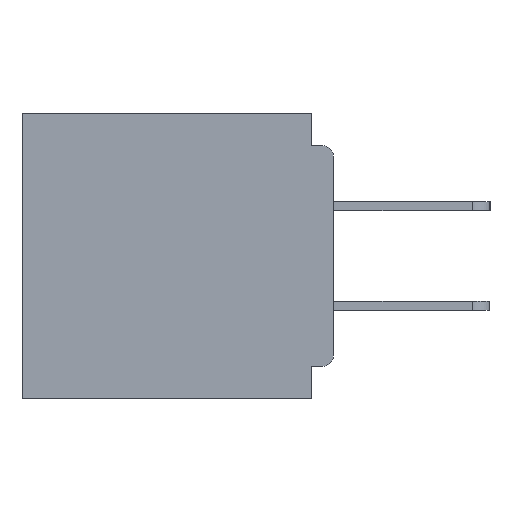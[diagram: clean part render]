
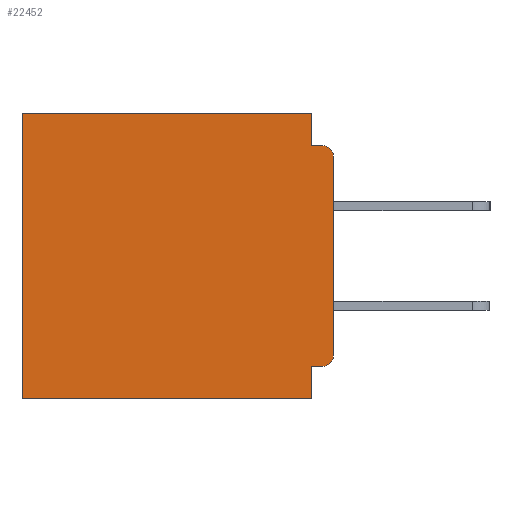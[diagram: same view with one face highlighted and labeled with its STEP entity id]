
A CAD part, left-side view. The second image highlights one B-rep face of the part: STEP entity #22452.
In plain terms, the highlighted planar face has unit normal (-1, 0, 0).
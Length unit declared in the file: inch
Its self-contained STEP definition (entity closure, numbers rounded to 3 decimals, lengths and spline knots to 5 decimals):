
#36 = VECTOR ( 'NONE', #17344, 39.37008 ) ;
#223 = CARTESIAN_POINT ( 'NONE',  ( 0.3, 0., -0.045 ) ) ;
#747 = CARTESIAN_POINT ( 'NONE',  ( 0.3, 0.015, -0.045 ) ) ;
#813 = CARTESIAN_POINT ( 'NONE',  ( 0.3, 0.437, 0. ) ) ;
#1583 = DIRECTION ( 'NONE',  ( 1., 0., 0. ) ) ;
#1776 = CARTESIAN_POINT ( 'NONE',  ( 0.3, 0.031, -0.4 ) ) ;
#1906 = CARTESIAN_POINT ( 'NONE',  ( 0.3, 0.015, -0.34 ) ) ;
#2342 = CARTESIAN_POINT ( 'NONE',  ( 0.3, 0., -0.4 ) ) ;
#3263 = LINE ( 'NONE', #28749, #34220 ) ;
#3384 = LINE ( 'NONE', #223, #34335 ) ;
#3968 = CARTESIAN_POINT ( 'NONE',  ( 0.3, 0., -0.34 ) ) ;
#4505 = ORIENTED_EDGE ( 'NONE', *, *, #13255, .T. ) ;
#4920 = DIRECTION ( 'NONE',  ( 0., 0., -1. ) ) ;
#5150 = ORIENTED_EDGE ( 'NONE', *, *, #34046, .F. ) ;
#5628 = ORIENTED_EDGE ( 'NONE', *, *, #17062, .F. ) ;
#6019 = ORIENTED_EDGE ( 'NONE', *, *, #33078, .F. ) ;
#6063 = LINE ( 'NONE', #6560, #13139 ) ;
#6167 = ORIENTED_EDGE ( 'NONE', *, *, #7210, .F. ) ;
#6421 = VERTEX_POINT ( 'NONE', #747 ) ;
#6560 = CARTESIAN_POINT ( 'NONE',  ( 0.3, 0., 0. ) ) ;
#6856 = VERTEX_POINT ( 'NONE', #31658 ) ;
#7210 = EDGE_CURVE ( 'NONE', #19645, #10606, #35064, .T. ) ;
#7676 = AXIS2_PLACEMENT_3D ( 'NONE', #1906, #22999, #4920 ) ;
#8122 = LINE ( 'NONE', #2342, #36 ) ;
#9248 = VERTEX_POINT ( 'NONE', #27892 ) ;
#10028 = LINE ( 'NONE', #26961, #17034 ) ;
#10606 = VERTEX_POINT ( 'NONE', #22914 ) ;
#11725 = VERTEX_POINT ( 'NONE', #3968 ) ;
#12478 = CARTESIAN_POINT ( 'NONE',  ( 0.3, 0.437, -0.4 ) ) ;
#12647 = EDGE_CURVE ( 'NONE', #25645, #32810, #30915, .T. ) ;
#13139 = VECTOR ( 'NONE', #18802, 39.37008 ) ;
#13255 = EDGE_CURVE ( 'NONE', #9248, #6421, #35891, .T. ) ;
#13530 = DIRECTION ( 'NONE',  ( -1., 0., 0. ) ) ;
#14939 = AXIS2_PLACEMENT_3D ( 'NONE', #31445, #13530, #34436 ) ;
#15056 = DIRECTION ( 'NONE',  ( 0., 0., -1. ) ) ;
#16601 = CARTESIAN_POINT ( 'NONE',  ( 0.3, 0.437, -0.4 ) ) ;
#17034 = VECTOR ( 'NONE', #15056, 39.37008 ) ;
#17062 = EDGE_CURVE ( 'NONE', #33677, #32810, #8122, .T. ) ;
#17344 = DIRECTION ( 'NONE',  ( 0., 1., 0. ) ) ;
#18188 = DIRECTION ( 'NONE',  ( 0., 1., 0. ) ) ;
#18802 = DIRECTION ( 'NONE',  ( 0., 1., 0. ) ) ;
#19645 = VERTEX_POINT ( 'NONE', #35760 ) ;
#19852 = DIRECTION ( 'NONE',  ( 0., 0., -1. ) ) ;
#20135 = ORIENTED_EDGE ( 'NONE', *, *, #12647, .T. ) ;
#20288 = ORIENTED_EDGE ( 'NONE', *, *, #25332, .T. ) ;
#20775 = FACE_OUTER_BOUND ( 'NONE', #38342, .T. ) ;
#21338 = DIRECTION ( 'NONE',  ( 0., -1., 0. ) ) ;
#22099 = EDGE_CURVE ( 'NONE', #9248, #11725, #10028, .T. ) ;
#22452 = ADVANCED_FACE ( 'NONE', ( #20775 ), #34476, .F. ) ;
#22471 = VERTEX_POINT ( 'NONE', #37245 ) ;
#22691 = DIRECTION ( 'NONE',  ( 0., 0., -1. ) ) ;
#22692 = DIRECTION ( 'NONE',  ( 0., 0., -1. ) ) ;
#22914 = CARTESIAN_POINT ( 'NONE',  ( 0.3, 0.031, -0.355 ) ) ;
#22999 = DIRECTION ( 'NONE',  ( -1., 0., 0. ) ) ;
#23131 = EDGE_CURVE ( 'NONE', #22471, #6856, #3263, .T. ) ;
#23277 = VECTOR ( 'NONE', #25716, 39.37008 ) ;
#25332 = EDGE_CURVE ( 'NONE', #19645, #11725, #30252, .T. ) ;
#25645 = VERTEX_POINT ( 'NONE', #813 ) ;
#25716 = DIRECTION ( 'NONE',  ( 0., 0., -1. ) ) ;
#26247 = VECTOR ( 'NONE', #18188, 39.37008 ) ;
#26961 = CARTESIAN_POINT ( 'NONE',  ( 0.3, 0., -0.4 ) ) ;
#27892 = CARTESIAN_POINT ( 'NONE',  ( 0.3, 0., -0.06 ) ) ;
#28749 = CARTESIAN_POINT ( 'NONE',  ( 0.3, 0.031, 0. ) ) ;
#30252 = CIRCLE ( 'NONE', #7676, 0.015 ) ;
#30297 = EDGE_CURVE ( 'NONE', #22471, #25645, #6063, .T. ) ;
#30915 = LINE ( 'NONE', #16601, #38660 ) ;
#31164 = LINE ( 'NONE', #1776, #23277 ) ;
#31445 = CARTESIAN_POINT ( 'NONE',  ( 0.3, 0.015, -0.06 ) ) ;
#31658 = CARTESIAN_POINT ( 'NONE',  ( 0.3, 0.031, -0.045 ) ) ;
#32735 = ORIENTED_EDGE ( 'NONE', *, *, #30297, .T. ) ;
#32810 = VERTEX_POINT ( 'NONE', #12478 ) ;
#33073 = CARTESIAN_POINT ( 'NONE',  ( 0.3, 0., -0.355 ) ) ;
#33078 = EDGE_CURVE ( 'NONE', #10606, #33677, #31164, .T. ) ;
#33511 = ORIENTED_EDGE ( 'NONE', *, *, #23131, .F. ) ;
#33677 = VERTEX_POINT ( 'NONE', #37387 ) ;
#34046 = EDGE_CURVE ( 'NONE', #6856, #6421, #3384, .T. ) ;
#34220 = VECTOR ( 'NONE', #19852, 39.37008 ) ;
#34335 = VECTOR ( 'NONE', #21338, 39.37008 ) ;
#34436 = DIRECTION ( 'NONE',  ( 0., 0., -1. ) ) ;
#34476 = PLANE ( 'NONE',  #35161 ) ;
#35064 = LINE ( 'NONE', #33073, #26247 ) ;
#35161 = AXIS2_PLACEMENT_3D ( 'NONE', #37372, #1583, #22692 ) ;
#35760 = CARTESIAN_POINT ( 'NONE',  ( 0.3, 0.015, -0.355 ) ) ;
#35891 = CIRCLE ( 'NONE', #14939, 0.015 ) ;
#37245 = CARTESIAN_POINT ( 'NONE',  ( 0.3, 0.031, 0. ) ) ;
#37372 = CARTESIAN_POINT ( 'NONE',  ( 0.3, 0., -0.4 ) ) ;
#37387 = CARTESIAN_POINT ( 'NONE',  ( 0.3, 0.031, -0.4 ) ) ;
#37798 = ORIENTED_EDGE ( 'NONE', *, *, #22099, .F. ) ;
#38342 = EDGE_LOOP ( 'NONE', ( #37798, #4505, #5150, #33511, #32735, #20135, #5628, #6019, #6167, #20288 ) ) ;
#38660 = VECTOR ( 'NONE', #22691, 39.37008 ) ;
